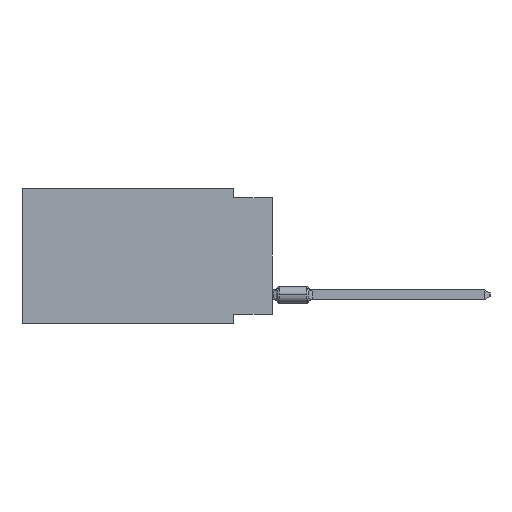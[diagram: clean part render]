
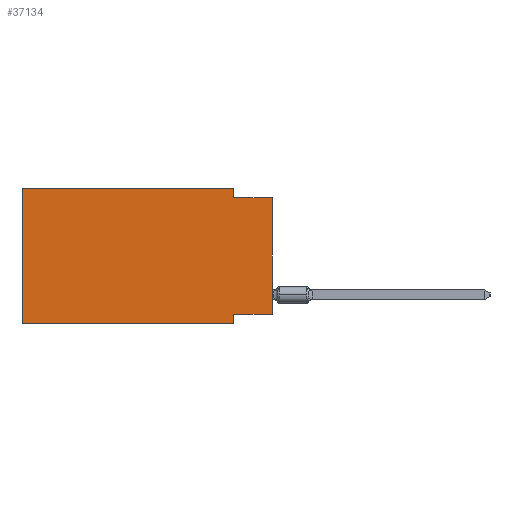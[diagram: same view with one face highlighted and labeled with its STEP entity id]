
A CAD part, left-side view. The second image highlights one B-rep face of the part: STEP entity #37134.
In plain terms, the highlighted planar face has unit normal (-1, 0, 0).
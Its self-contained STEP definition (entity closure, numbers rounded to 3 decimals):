
#765 = CARTESIAN_POINT ( 'NONE',  ( 0., 2.54, -8.255 ) ) ;
#981 = VERTEX_POINT ( 'NONE', #13198 ) ;
#2541 = VECTOR ( 'NONE', #41332, 1000. ) ;
#3444 = CARTESIAN_POINT ( 'NONE',  ( 0., 16.383, 0. ) ) ;
#4189 = CARTESIAN_POINT ( 'NONE',  ( 0., 2.54, -0.635 ) ) ;
#4195 = EDGE_CURVE ( 'NONE', #7436, #41232, #44624, .T. ) ;
#7424 = DIRECTION ( 'NONE',  ( 0., -1., 0. ) ) ;
#7436 = VERTEX_POINT ( 'NONE', #4189 ) ;
#9971 = ORIENTED_EDGE ( 'NONE', *, *, #29709, .F. ) ;
#10014 = CARTESIAN_POINT ( 'NONE',  ( 0., 0., 0. ) ) ;
#10762 = VERTEX_POINT ( 'NONE', #765 ) ;
#10797 = CARTESIAN_POINT ( 'NONE',  ( 0., 16.383, 0. ) ) ;
#12281 = CARTESIAN_POINT ( 'NONE',  ( 0., 2.54, 0. ) ) ;
#12340 = EDGE_CURVE ( 'NONE', #32309, #12889, #14748, .T. ) ;
#12543 = VECTOR ( 'NONE', #36351, 1000. ) ;
#12889 = VERTEX_POINT ( 'NONE', #12907 ) ;
#12907 = CARTESIAN_POINT ( 'NONE',  ( 0., 2.54, 0. ) ) ;
#13198 = CARTESIAN_POINT ( 'NONE',  ( 0., 0., -8.255 ) ) ;
#13287 = CARTESIAN_POINT ( 'NONE',  ( 0., 0., -8.255 ) ) ;
#13701 = EDGE_CURVE ( 'NONE', #32808, #32309, #48580, .T. ) ;
#14091 = VECTOR ( 'NONE', #44232, 1000. ) ;
#14662 = ORIENTED_EDGE ( 'NONE', *, *, #13701, .F. ) ;
#14748 = LINE ( 'NONE', #10797, #2541 ) ;
#15500 = DIRECTION ( 'NONE',  ( 0., -1., 0. ) ) ;
#15602 = FACE_OUTER_BOUND ( 'NONE', #45397, .T. ) ;
#15756 = LINE ( 'NONE', #34881, #42608 ) ;
#19023 = VERTEX_POINT ( 'NONE', #32809 ) ;
#20309 = CARTESIAN_POINT ( 'NONE',  ( 0., 16.383, 0. ) ) ;
#20494 = VECTOR ( 'NONE', #41402, 1000. ) ;
#21249 = CARTESIAN_POINT ( 'NONE',  ( 0., 0., -0.635 ) ) ;
#22740 = ORIENTED_EDGE ( 'NONE', *, *, #46485, .F. ) ;
#23837 = EDGE_CURVE ( 'NONE', #10762, #19023, #15756, .T. ) ;
#23995 = EDGE_CURVE ( 'NONE', #981, #41232, #43988, .T. ) ;
#24054 = DIRECTION ( 'NONE',  ( 0., 0., -1. ) ) ;
#24347 = VECTOR ( 'NONE', #15500, 1000. ) ;
#24674 = LINE ( 'NONE', #12281, #32432 ) ;
#27786 = PLANE ( 'NONE',  #32572 ) ;
#28867 = ORIENTED_EDGE ( 'NONE', *, *, #12340, .F. ) ;
#29709 = EDGE_CURVE ( 'NONE', #12889, #7436, #24674, .T. ) ;
#32309 = VERTEX_POINT ( 'NONE', #47889 ) ;
#32432 = VECTOR ( 'NONE', #47181, 1000. ) ;
#32572 = AXIS2_PLACEMENT_3D ( 'NONE', #20309, #42903, #24054 ) ;
#32808 = VERTEX_POINT ( 'NONE', #37429 ) ;
#32809 = CARTESIAN_POINT ( 'NONE',  ( 0., 2.54, -8.89 ) ) ;
#33243 = ORIENTED_EDGE ( 'NONE', *, *, #39637, .T. ) ;
#34386 = DIRECTION ( 'NONE',  ( 0., 0., -1. ) ) ;
#34881 = CARTESIAN_POINT ( 'NONE',  ( 0., 2.54, -8.89 ) ) ;
#36351 = DIRECTION ( 'NONE',  ( 0., 1., 0. ) ) ;
#37134 = ADVANCED_FACE ( 'NONE', ( #15602 ), #27786, .F. ) ;
#37429 = CARTESIAN_POINT ( 'NONE',  ( 0., 16.383, -8.89 ) ) ;
#37440 = CARTESIAN_POINT ( 'NONE',  ( 0., 0., -0.635 ) ) ;
#39064 = ORIENTED_EDGE ( 'NONE', *, *, #23837, .F. ) ;
#39637 = EDGE_CURVE ( 'NONE', #32808, #19023, #48993, .T. ) ;
#39946 = ORIENTED_EDGE ( 'NONE', *, *, #23995, .T. ) ;
#41232 = VERTEX_POINT ( 'NONE', #21249 ) ;
#41332 = DIRECTION ( 'NONE',  ( 0., -1., 0. ) ) ;
#41402 = DIRECTION ( 'NONE',  ( 0., 0., 1. ) ) ;
#41806 = CARTESIAN_POINT ( 'NONE',  ( 0., 16.383, -8.89 ) ) ;
#42608 = VECTOR ( 'NONE', #34386, 1000. ) ;
#42903 = DIRECTION ( 'NONE',  ( 1., 0., 0. ) ) ;
#43988 = LINE ( 'NONE', #10014, #14091 ) ;
#44232 = DIRECTION ( 'NONE',  ( 0., 0., 1. ) ) ;
#44624 = LINE ( 'NONE', #37440, #45126 ) ;
#45126 = VECTOR ( 'NONE', #7424, 1000. ) ;
#45397 = EDGE_LOOP ( 'NONE', ( #39946, #46454, #9971, #28867, #14662, #33243, #39064, #22740 ) ) ;
#46454 = ORIENTED_EDGE ( 'NONE', *, *, #4195, .F. ) ;
#46485 = EDGE_CURVE ( 'NONE', #981, #10762, #47241, .T. ) ;
#47181 = DIRECTION ( 'NONE',  ( 0., 0., -1. ) ) ;
#47241 = LINE ( 'NONE', #13287, #12543 ) ;
#47889 = CARTESIAN_POINT ( 'NONE',  ( 0., 16.383, 0. ) ) ;
#48580 = LINE ( 'NONE', #3444, #20494 ) ;
#48993 = LINE ( 'NONE', #41806, #24347 ) ;
